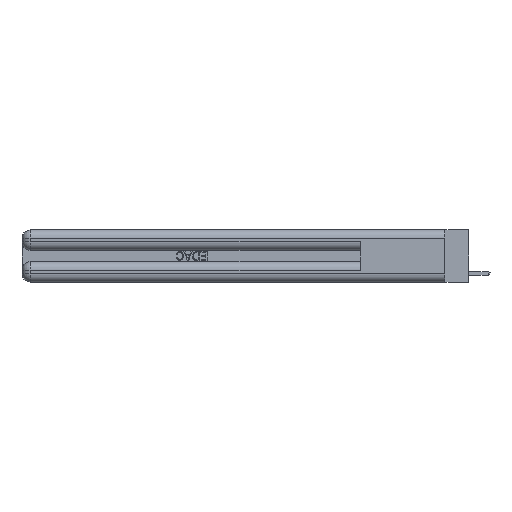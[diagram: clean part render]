
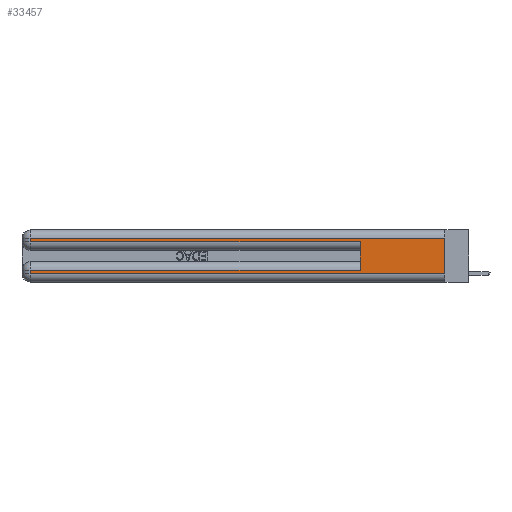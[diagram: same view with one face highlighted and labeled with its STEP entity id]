
A CAD part, left-side view. The second image highlights one B-rep face of the part: STEP entity #33457.
In plain terms, the highlighted planar face has unit normal (-1, 0, 0).
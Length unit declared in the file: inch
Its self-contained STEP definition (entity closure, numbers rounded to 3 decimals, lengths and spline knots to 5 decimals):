
#64 = LINE ( 'NONE', #16623, #27402 ) ;
#1037 = PLANE ( 'NONE',  #22124 ) ;
#1368 = VECTOR ( 'NONE', #14501, 39.37008 ) ;
#1577 = VECTOR ( 'NONE', #17097, 39.37008 ) ;
#1654 = ORIENTED_EDGE ( 'NONE', *, *, #5769, .T. ) ;
#2455 = CARTESIAN_POINT ( 'NONE',  ( 0., 0., 0.06 ) ) ;
#2706 = VECTOR ( 'NONE', #21749, 39.37008 ) ;
#2734 = CARTESIAN_POINT ( 'NONE',  ( 0., 2.94, 0.37 ) ) ;
#3152 = CARTESIAN_POINT ( 'NONE',  ( 0., 2.94, 0.37 ) ) ;
#3445 = DIRECTION ( 'NONE',  ( 1., 0., 0. ) ) ;
#3502 = CARTESIAN_POINT ( 'NONE',  ( 0., 0.6, 0.085 ) ) ;
#5029 = CARTESIAN_POINT ( 'NONE',  ( 0., 2.94, 0.285 ) ) ;
#5456 = EDGE_LOOP ( 'NONE', ( #16486, #28363, #33238, #1654, #6029, #30909, #14610, #16293 ) ) ;
#5514 = CARTESIAN_POINT ( 'NONE',  ( 0., 0., 0.37 ) ) ;
#5769 = EDGE_CURVE ( 'NONE', #17311, #11376, #10212, .T. ) ;
#5877 = VERTEX_POINT ( 'NONE', #22577 ) ;
#6029 = ORIENTED_EDGE ( 'NONE', *, *, #19086, .F. ) ;
#7429 = DIRECTION ( 'NONE',  ( 0., 1., 0. ) ) ;
#8076 = LINE ( 'NONE', #3152, #2706 ) ;
#9393 = EDGE_CURVE ( 'NONE', #15000, #17311, #24887, .T. ) ;
#9829 = CARTESIAN_POINT ( 'NONE',  ( 0., 0., 0.31 ) ) ;
#10212 = LINE ( 'NONE', #14227, #1577 ) ;
#11376 = VERTEX_POINT ( 'NONE', #17253 ) ;
#11676 = DIRECTION ( 'NONE',  ( 0., -1., 0. ) ) ;
#12086 = CARTESIAN_POINT ( 'NONE',  ( 0., 0., 0.31 ) ) ;
#13003 = VECTOR ( 'NONE', #7429, 39.37008 ) ;
#14019 = EDGE_CURVE ( 'NONE', #24058, #15000, #29207, .T. ) ;
#14227 = CARTESIAN_POINT ( 'NONE',  ( 0., 0., 0.285 ) ) ;
#14501 = DIRECTION ( 'NONE',  ( 0., 0., 1. ) ) ;
#14610 = ORIENTED_EDGE ( 'NONE', *, *, #24127, .T. ) ;
#15000 = VERTEX_POINT ( 'NONE', #25187 ) ;
#15598 = VECTOR ( 'NONE', #16944, 39.37008 ) ;
#16293 = ORIENTED_EDGE ( 'NONE', *, *, #27409, .T. ) ;
#16486 = ORIENTED_EDGE ( 'NONE', *, *, #22496, .F. ) ;
#16623 = CARTESIAN_POINT ( 'NONE',  ( 0., 0., 0.06 ) ) ;
#16944 = DIRECTION ( 'NONE',  ( 0., 1., 0. ) ) ;
#17097 = DIRECTION ( 'NONE',  ( 0., -1., 0. ) ) ;
#17253 = CARTESIAN_POINT ( 'NONE',  ( 0., 0.6, 0.285 ) ) ;
#17261 = LINE ( 'NONE', #5514, #26027 ) ;
#17311 = VERTEX_POINT ( 'NONE', #5029 ) ;
#17675 = LINE ( 'NONE', #20097, #15598 ) ;
#17744 = VERTEX_POINT ( 'NONE', #2455 ) ;
#18192 = DIRECTION ( 'NONE',  ( 0., 0., -1. ) ) ;
#18496 = CARTESIAN_POINT ( 'NONE',  ( 0., 2.94, 0.085 ) ) ;
#19086 = EDGE_CURVE ( 'NONE', #27353, #11376, #21208, .T. ) ;
#19273 = FACE_OUTER_BOUND ( 'NONE', #5456, .T. ) ;
#20097 = CARTESIAN_POINT ( 'NONE',  ( 0., 0., 0.085 ) ) ;
#21208 = LINE ( 'NONE', #32874, #1368 ) ;
#21749 = DIRECTION ( 'NONE',  ( 0., 0., -1. ) ) ;
#22124 = AXIS2_PLACEMENT_3D ( 'NONE', #27321, #3445, #32988 ) ;
#22496 = EDGE_CURVE ( 'NONE', #24058, #17744, #17261, .T. ) ;
#22577 = CARTESIAN_POINT ( 'NONE',  ( 0., 2.94, 0.06 ) ) ;
#23192 = VECTOR ( 'NONE', #18192, 39.37008 ) ;
#23303 = VERTEX_POINT ( 'NONE', #18496 ) ;
#24058 = VERTEX_POINT ( 'NONE', #9829 ) ;
#24127 = EDGE_CURVE ( 'NONE', #23303, #5877, #8076, .T. ) ;
#24887 = LINE ( 'NONE', #2734, #23192 ) ;
#25187 = CARTESIAN_POINT ( 'NONE',  ( 0., 2.94, 0.31 ) ) ;
#26027 = VECTOR ( 'NONE', #29401, 39.37008 ) ;
#27321 = CARTESIAN_POINT ( 'NONE',  ( 0., 0., 0.37 ) ) ;
#27353 = VERTEX_POINT ( 'NONE', #3502 ) ;
#27402 = VECTOR ( 'NONE', #11676, 39.37008 ) ;
#27409 = EDGE_CURVE ( 'NONE', #5877, #17744, #64, .T. ) ;
#28363 = ORIENTED_EDGE ( 'NONE', *, *, #14019, .T. ) ;
#29207 = LINE ( 'NONE', #12086, #13003 ) ;
#29401 = DIRECTION ( 'NONE',  ( 0., 0., -1. ) ) ;
#30909 = ORIENTED_EDGE ( 'NONE', *, *, #32282, .T. ) ;
#32282 = EDGE_CURVE ( 'NONE', #27353, #23303, #17675, .T. ) ;
#32874 = CARTESIAN_POINT ( 'NONE',  ( 0., 0.6, 0.145 ) ) ;
#32988 = DIRECTION ( 'NONE',  ( 0., 0., -1. ) ) ;
#33238 = ORIENTED_EDGE ( 'NONE', *, *, #9393, .T. ) ;
#33457 = ADVANCED_FACE ( 'NONE', ( #19273 ), #1037, .F. ) ;
